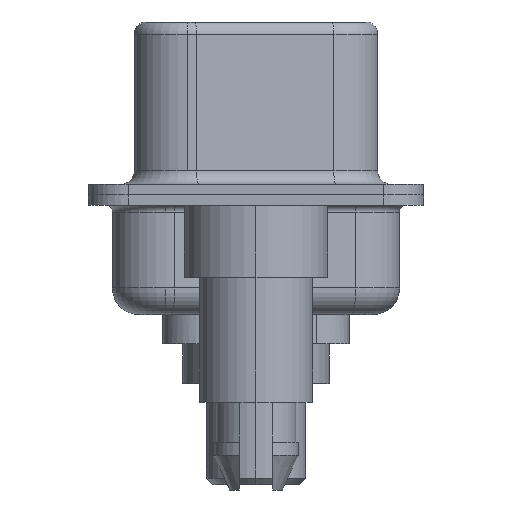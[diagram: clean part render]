
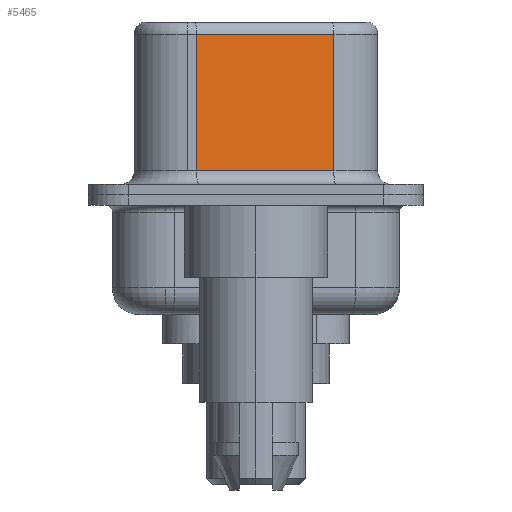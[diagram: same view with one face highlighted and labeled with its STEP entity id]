
A CAD part, left-side view. The second image highlights one B-rep face of the part: STEP entity #5465.
In plain terms, the highlighted planar face has unit normal (-0.985, -0.174, 0).
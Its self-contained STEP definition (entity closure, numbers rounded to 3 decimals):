
#596 = LINE ( 'NONE', #2057, #17038 ) ;
#731 = LINE ( 'NONE', #17493, #11929 ) ;
#1568 = VECTOR ( 'NONE', #13353, 1000. ) ;
#1759 = EDGE_CURVE ( 'NONE', #5101, #14279, #596, .T. ) ;
#2057 = CARTESIAN_POINT ( 'NONE',  ( 4.565, -2.927, 6.52 ) ) ;
#2167 = CARTESIAN_POINT ( 'NONE',  ( 3.655, 2.233, 6.02 ) ) ;
#2272 = EDGE_CURVE ( 'NONE', #5101, #9973, #13268, .T. ) ;
#3051 = EDGE_CURVE ( 'NONE', #9973, #15756, #4416, .T. ) ;
#3228 = DIRECTION ( 'NONE',  ( 0.174, -0.985, 0. ) ) ;
#4143 = ORIENTED_EDGE ( 'NONE', *, *, #20594, .T. ) ;
#4416 = LINE ( 'NONE', #14436, #12331 ) ;
#4789 = ORIENTED_EDGE ( 'NONE', *, *, #3051, .T. ) ;
#4958 = DIRECTION ( 'NONE',  ( 0.985, 0.174, 0. ) ) ;
#5101 = VERTEX_POINT ( 'NONE', #13926 ) ;
#5465 = ADVANCED_FACE ( 'NONE', ( #19744 ), #20590, .F. ) ;
#6004 = DIRECTION ( 'NONE',  ( -0.174, 0.985, 0. ) ) ;
#6652 = DIRECTION ( 'NONE',  ( 0., 0., -1. ) ) ;
#8520 = DIRECTION ( 'NONE',  ( 0., 0., -1. ) ) ;
#9973 = VERTEX_POINT ( 'NONE', #2167 ) ;
#11581 = AXIS2_PLACEMENT_3D ( 'NONE', #12276, #4958, #6004 ) ;
#11929 = VECTOR ( 'NONE', #3228, 1000. ) ;
#12077 = CARTESIAN_POINT ( 'NONE',  ( 3.655, 2.233, 0.9 ) ) ;
#12276 = CARTESIAN_POINT ( 'NONE',  ( 4.565, -2.927, 6.52 ) ) ;
#12331 = VECTOR ( 'NONE', #6652, 1000. ) ;
#13268 = LINE ( 'NONE', #16335, #1568 ) ;
#13353 = DIRECTION ( 'NONE',  ( -0.174, 0.985, 0. ) ) ;
#13926 = CARTESIAN_POINT ( 'NONE',  ( 4.565, -2.927, 6.02 ) ) ;
#14279 = VERTEX_POINT ( 'NONE', #19183 ) ;
#14436 = CARTESIAN_POINT ( 'NONE',  ( 3.655, 2.233, 6.52 ) ) ;
#15756 = VERTEX_POINT ( 'NONE', #12077 ) ;
#16335 = CARTESIAN_POINT ( 'NONE',  ( 4.565, -2.927, 6.02 ) ) ;
#16438 = ORIENTED_EDGE ( 'NONE', *, *, #2272, .T. ) ;
#16995 = ORIENTED_EDGE ( 'NONE', *, *, #1759, .F. ) ;
#17038 = VECTOR ( 'NONE', #8520, 1000. ) ;
#17493 = CARTESIAN_POINT ( 'NONE',  ( 4.565, -2.927, 0.9 ) ) ;
#18536 = EDGE_LOOP ( 'NONE', ( #16995, #16438, #4789, #4143 ) ) ;
#19183 = CARTESIAN_POINT ( 'NONE',  ( 4.565, -2.927, 0.9 ) ) ;
#19744 = FACE_OUTER_BOUND ( 'NONE', #18536, .T. ) ;
#20590 = PLANE ( 'NONE',  #11581 ) ;
#20594 = EDGE_CURVE ( 'NONE', #15756, #14279, #731, .T. ) ;
